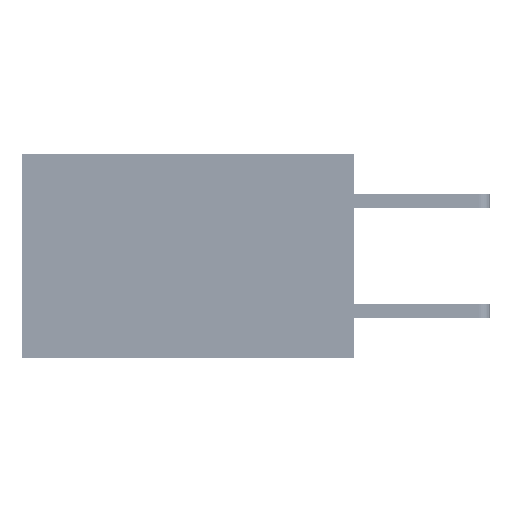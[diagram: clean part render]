
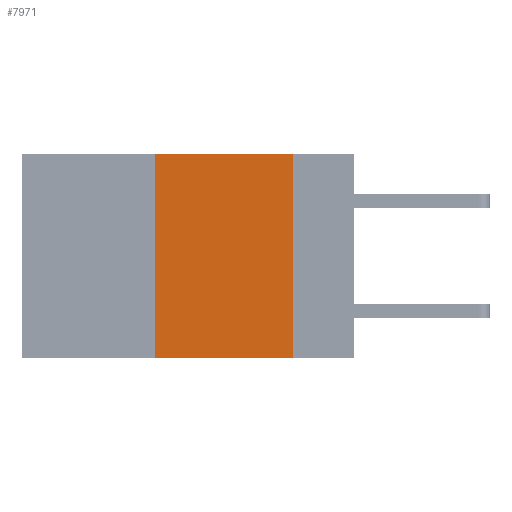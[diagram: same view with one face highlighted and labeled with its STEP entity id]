
A CAD part, left-side view. The second image highlights one B-rep face of the part: STEP entity #7971.
In plain terms, the highlighted planar face has unit normal (-1, 0, 0).
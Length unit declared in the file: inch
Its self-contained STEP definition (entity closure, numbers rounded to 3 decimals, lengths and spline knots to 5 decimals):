
#2073 = VECTOR ( 'NONE', #35586, 39.37008 ) ;
#3027 = EDGE_CURVE ( 'NONE', #10858, #28746, #47810, .T. ) ;
#6209 = EDGE_CURVE ( 'NONE', #21084, #28746, #44711, .T. ) ;
#7019 = EDGE_CURVE ( 'NONE', #18039, #10858, #40124, .T. ) ;
#7971 = ADVANCED_FACE ( 'NONE', ( #18347 ), #43696, .F. ) ;
#8008 = AXIS2_PLACEMENT_3D ( 'NONE', #33355, #40492, #10737 ) ;
#10737 = DIRECTION ( 'NONE',  ( 0., 0., -1. ) ) ;
#10858 = VERTEX_POINT ( 'NONE', #25720 ) ;
#11998 = EDGE_CURVE ( 'NONE', #21084, #18039, #38789, .T. ) ;
#13566 = VECTOR ( 'NONE', #16094, 39.37008 ) ;
#16094 = DIRECTION ( 'NONE',  ( 0., -1., 0. ) ) ;
#16196 = CARTESIAN_POINT ( 'NONE',  ( 0., 0.36, 0. ) ) ;
#18039 = VERTEX_POINT ( 'NONE', #16196 ) ;
#18347 = FACE_OUTER_BOUND ( 'NONE', #43154, .T. ) ;
#19860 = VECTOR ( 'NONE', #32922, 39.37008 ) ;
#20559 = CARTESIAN_POINT ( 'NONE',  ( 0., 0.36, -0.37 ) ) ;
#21084 = VERTEX_POINT ( 'NONE', #20559 ) ;
#22692 = CARTESIAN_POINT ( 'NONE',  ( 0., 0.11, 0. ) ) ;
#25720 = CARTESIAN_POINT ( 'NONE',  ( 0., 0.11, 0. ) ) ;
#28746 = VERTEX_POINT ( 'NONE', #46995 ) ;
#28873 = ORIENTED_EDGE ( 'NONE', *, *, #3027, .F. ) ;
#32922 = DIRECTION ( 'NONE',  ( 0., -1., 0. ) ) ;
#33355 = CARTESIAN_POINT ( 'NONE',  ( 0., 0.6, 0. ) ) ;
#33646 = CARTESIAN_POINT ( 'NONE',  ( 0., 0.6, -0.37 ) ) ;
#34544 = ORIENTED_EDGE ( 'NONE', *, *, #7019, .F. ) ;
#34817 = ORIENTED_EDGE ( 'NONE', *, *, #11998, .F. ) ;
#35586 = DIRECTION ( 'NONE',  ( 0., 0., 1. ) ) ;
#38789 = LINE ( 'NONE', #42954, #2073 ) ;
#39215 = ORIENTED_EDGE ( 'NONE', *, *, #6209, .T. ) ;
#40124 = LINE ( 'NONE', #47730, #13566 ) ;
#40492 = DIRECTION ( 'NONE',  ( 1., 0., 0. ) ) ;
#42954 = CARTESIAN_POINT ( 'NONE',  ( 0., 0.36, 0. ) ) ;
#43154 = EDGE_LOOP ( 'NONE', ( #28873, #34544, #34817, #39215 ) ) ;
#43696 = PLANE ( 'NONE',  #8008 ) ;
#44711 = LINE ( 'NONE', #33646, #19860 ) ;
#46995 = CARTESIAN_POINT ( 'NONE',  ( 0., 0.11, -0.37 ) ) ;
#47119 = VECTOR ( 'NONE', #48052, 39.37008 ) ;
#47730 = CARTESIAN_POINT ( 'NONE',  ( 0., 0.6, 0. ) ) ;
#47810 = LINE ( 'NONE', #22692, #47119 ) ;
#48052 = DIRECTION ( 'NONE',  ( 0., 0., -1. ) ) ;
